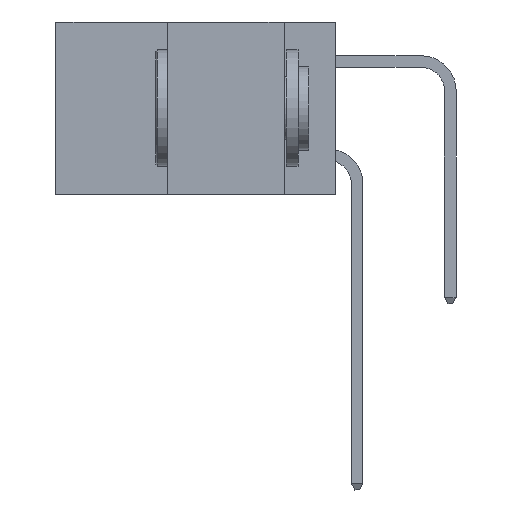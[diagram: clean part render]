
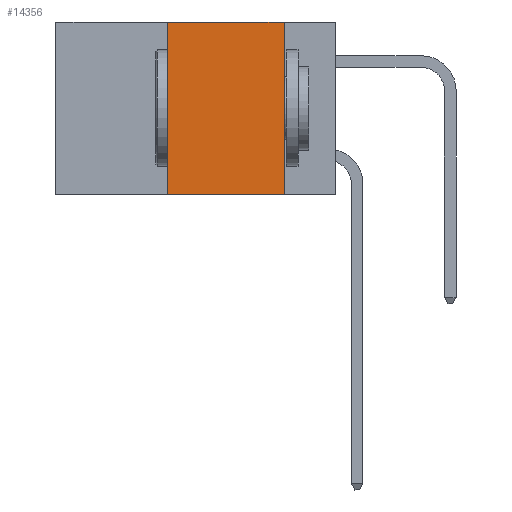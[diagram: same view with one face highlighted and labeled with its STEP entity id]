
A CAD part, left-side view. The second image highlights one B-rep face of the part: STEP entity #14356.
In plain terms, the highlighted planar face has unit normal (-1, 0, 0).
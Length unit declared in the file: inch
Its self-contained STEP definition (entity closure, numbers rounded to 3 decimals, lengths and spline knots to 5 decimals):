
#1115 = DIRECTION ( 'NONE',  ( 0., 0., 1. ) ) ;
#1369 = VERTEX_POINT ( 'NONE', #21855 ) ;
#1499 = VERTEX_POINT ( 'NONE', #18387 ) ;
#1797 = DIRECTION ( 'NONE',  ( 0., -1., 0. ) ) ;
#1987 = VECTOR ( 'NONE', #1115, 39.37008 ) ;
#2578 = LINE ( 'NONE', #8853, #1987 ) ;
#3305 = AXIS2_PLACEMENT_3D ( 'NONE', #15502, #17345, #6082 ) ;
#4197 = PLANE ( 'NONE',  #3305 ) ;
#4271 = LINE ( 'NONE', #19753, #23508 ) ;
#5500 = ORIENTED_EDGE ( 'NONE', *, *, #15200, .F. ) ;
#6082 = DIRECTION ( 'NONE',  ( 0., 0., -1. ) ) ;
#8583 = VERTEX_POINT ( 'NONE', #16939 ) ;
#8831 = LINE ( 'NONE', #21953, #12730 ) ;
#8853 = CARTESIAN_POINT ( 'NONE',  ( 0., 0.36, 0. ) ) ;
#9341 = ORIENTED_EDGE ( 'NONE', *, *, #19776, .F. ) ;
#9569 = LINE ( 'NONE', #20625, #15178 ) ;
#11608 = EDGE_CURVE ( 'NONE', #1369, #8583, #9569, .T. ) ;
#12365 = ORIENTED_EDGE ( 'NONE', *, *, #14043, .T. ) ;
#12377 = DIRECTION ( 'NONE',  ( 0., 0., -1. ) ) ;
#12730 = VECTOR ( 'NONE', #23743, 39.37008 ) ;
#14043 = EDGE_CURVE ( 'NONE', #18961, #1499, #8831, .T. ) ;
#14356 = ADVANCED_FACE ( 'NONE', ( #20517 ), #4197, .F. ) ;
#15178 = VECTOR ( 'NONE', #1797, 39.37008 ) ;
#15200 = EDGE_CURVE ( 'NONE', #18961, #1369, #2578, .T. ) ;
#15502 = CARTESIAN_POINT ( 'NONE',  ( 0., 0.6, 0. ) ) ;
#16939 = CARTESIAN_POINT ( 'NONE',  ( 0., 0.11, 0. ) ) ;
#17345 = DIRECTION ( 'NONE',  ( 1., 0., 0. ) ) ;
#18387 = CARTESIAN_POINT ( 'NONE',  ( 0., 0.11, -0.37 ) ) ;
#18961 = VERTEX_POINT ( 'NONE', #21244 ) ;
#19753 = CARTESIAN_POINT ( 'NONE',  ( 0., 0.11, 0. ) ) ;
#19776 = EDGE_CURVE ( 'NONE', #8583, #1499, #4271, .T. ) ;
#19873 = ORIENTED_EDGE ( 'NONE', *, *, #11608, .F. ) ;
#20517 = FACE_OUTER_BOUND ( 'NONE', #21027, .T. ) ;
#20625 = CARTESIAN_POINT ( 'NONE',  ( 0., 0.6, 0. ) ) ;
#21027 = EDGE_LOOP ( 'NONE', ( #9341, #19873, #5500, #12365 ) ) ;
#21244 = CARTESIAN_POINT ( 'NONE',  ( 0., 0.36, -0.37 ) ) ;
#21855 = CARTESIAN_POINT ( 'NONE',  ( 0., 0.36, 0. ) ) ;
#21953 = CARTESIAN_POINT ( 'NONE',  ( 0., 0.6, -0.37 ) ) ;
#23508 = VECTOR ( 'NONE', #12377, 39.37008 ) ;
#23743 = DIRECTION ( 'NONE',  ( 0., -1., 0. ) ) ;
